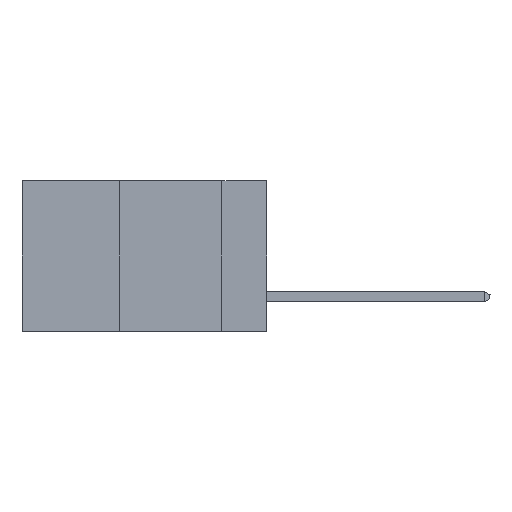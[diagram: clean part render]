
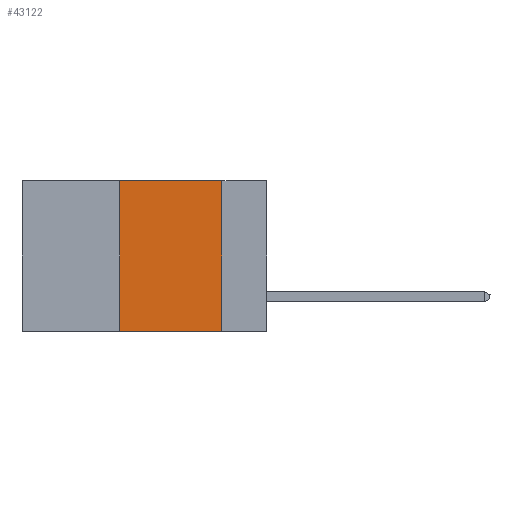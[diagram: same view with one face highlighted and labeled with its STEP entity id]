
A CAD part, left-side view. The second image highlights one B-rep face of the part: STEP entity #43122.
In plain terms, the highlighted planar face has unit normal (-1, 0, 0).
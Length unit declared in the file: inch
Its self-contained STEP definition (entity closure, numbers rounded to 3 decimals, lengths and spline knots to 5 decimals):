
#1979 = DIRECTION ( 'NONE',  ( 0., -1., 0. ) ) ;
#2480 = LINE ( 'NONE', #32618, #33443 ) ;
#3206 = CARTESIAN_POINT ( 'NONE',  ( 0., 0.36, 0. ) ) ;
#4150 = CARTESIAN_POINT ( 'NONE',  ( 0., 0.6, 0. ) ) ;
#5533 = CARTESIAN_POINT ( 'NONE',  ( 0., 0.36, 0. ) ) ;
#6635 = CARTESIAN_POINT ( 'NONE',  ( 0., 0.11, 0. ) ) ;
#7619 = DIRECTION ( 'NONE',  ( 1., 0., 0. ) ) ;
#8825 = DIRECTION ( 'NONE',  ( 0., 0., 1. ) ) ;
#8853 = DIRECTION ( 'NONE',  ( 0., -1., 0. ) ) ;
#9039 = DIRECTION ( 'NONE',  ( 0., 0., -1. ) ) ;
#10439 = EDGE_CURVE ( 'NONE', #36305, #40484, #2480, .T. ) ;
#10580 = VECTOR ( 'NONE', #8825, 39.37008 ) ;
#11509 = LINE ( 'NONE', #30437, #39054 ) ;
#13065 = ORIENTED_EDGE ( 'NONE', *, *, #14368, .T. ) ;
#13932 = ORIENTED_EDGE ( 'NONE', *, *, #10439, .F. ) ;
#14368 = EDGE_CURVE ( 'NONE', #15898, #35024, #11509, .T. ) ;
#14566 = VECTOR ( 'NONE', #9039, 39.37008 ) ;
#15898 = VERTEX_POINT ( 'NONE', #26873 ) ;
#17674 = EDGE_CURVE ( 'NONE', #40484, #35024, #44382, .T. ) ;
#17899 = LINE ( 'NONE', #5533, #10580 ) ;
#18010 = PLANE ( 'NONE',  #39910 ) ;
#26873 = CARTESIAN_POINT ( 'NONE',  ( 0., 0.36, -0.37 ) ) ;
#30437 = CARTESIAN_POINT ( 'NONE',  ( 0., 0.6, -0.37 ) ) ;
#31081 = EDGE_LOOP ( 'NONE', ( #42180, #13932, #37126, #13065 ) ) ;
#31635 = CARTESIAN_POINT ( 'NONE',  ( 0., 0.11, -0.37 ) ) ;
#32618 = CARTESIAN_POINT ( 'NONE',  ( 0., 0.6, 0. ) ) ;
#33443 = VECTOR ( 'NONE', #1979, 39.37008 ) ;
#33899 = FACE_OUTER_BOUND ( 'NONE', #31081, .T. ) ;
#35024 = VERTEX_POINT ( 'NONE', #31635 ) ;
#36305 = VERTEX_POINT ( 'NONE', #3206 ) ;
#36599 = EDGE_CURVE ( 'NONE', #15898, #36305, #17899, .T. ) ;
#37126 = ORIENTED_EDGE ( 'NONE', *, *, #36599, .F. ) ;
#39054 = VECTOR ( 'NONE', #8853, 39.37008 ) ;
#39910 = AXIS2_PLACEMENT_3D ( 'NONE', #4150, #7619, #40134 ) ;
#40134 = DIRECTION ( 'NONE',  ( 0., 0., -1. ) ) ;
#40484 = VERTEX_POINT ( 'NONE', #6635 ) ;
#42180 = ORIENTED_EDGE ( 'NONE', *, *, #17674, .F. ) ;
#43122 = ADVANCED_FACE ( 'NONE', ( #33899 ), #18010, .F. ) ;
#44382 = LINE ( 'NONE', #45231, #14566 ) ;
#45231 = CARTESIAN_POINT ( 'NONE',  ( 0., 0.11, 0. ) ) ;
